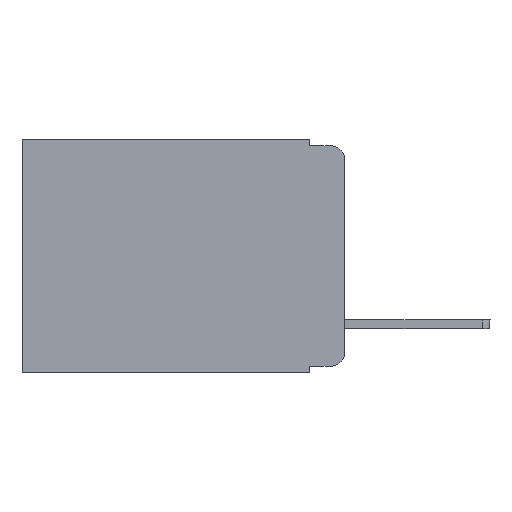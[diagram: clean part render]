
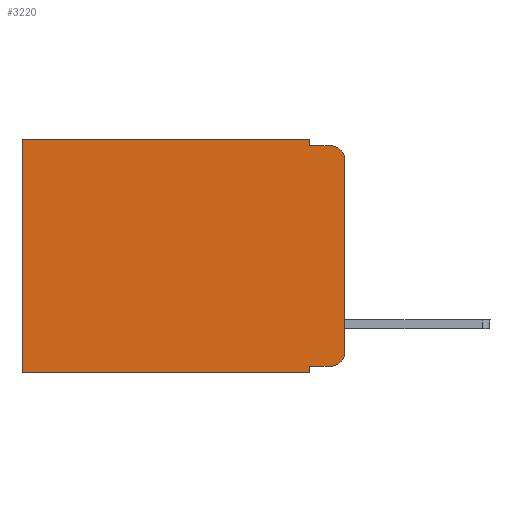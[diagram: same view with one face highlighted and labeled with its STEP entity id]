
A CAD part, left-side view. The second image highlights one B-rep face of the part: STEP entity #3220.
In plain terms, the highlighted planar face has unit normal (-1, 0, 0).
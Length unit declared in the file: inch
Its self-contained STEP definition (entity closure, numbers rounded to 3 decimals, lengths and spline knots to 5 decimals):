
#74 = VERTEX_POINT ( 'NONE', #2436 ) ;
#82 = ORIENTED_EDGE ( 'NONE', *, *, #1226, .T. ) ;
#198 = VERTEX_POINT ( 'NONE', #4855 ) ;
#212 = CARTESIAN_POINT ( 'NONE',  ( 0.298, 0., 0. ) ) ;
#234 = CIRCLE ( 'NONE', #6857, 0.02 ) ;
#612 = AXIS2_PLACEMENT_3D ( 'NONE', #3155, #5380, #3840 ) ;
#666 = EDGE_CURVE ( 'NONE', #4976, #74, #4478, .T. ) ;
#741 = EDGE_CURVE ( 'NONE', #7621, #8186, #6420, .T. ) ;
#754 = EDGE_CURVE ( 'NONE', #7621, #198, #1548, .T. ) ;
#815 = PLANE ( 'NONE',  #612 ) ;
#822 = VECTOR ( 'NONE', #1007, 39.37008 ) ;
#1007 = DIRECTION ( 'NONE',  ( 0., 0., -1. ) ) ;
#1194 = VECTOR ( 'NONE', #4541, 39.37008 ) ;
#1226 = EDGE_CURVE ( 'NONE', #8186, #9076, #8198, .T. ) ;
#1530 = VERTEX_POINT ( 'NONE', #3482 ) ;
#1548 = LINE ( 'NONE', #5641, #822 ) ;
#1569 = DIRECTION ( 'NONE',  ( 0., 0., -1. ) ) ;
#1584 = ORIENTED_EDGE ( 'NONE', *, *, #666, .F. ) ;
#1820 = EDGE_CURVE ( 'NONE', #5080, #1530, #2752, .T. ) ;
#1843 = VECTOR ( 'NONE', #6086, 39.37008 ) ;
#2134 = FACE_OUTER_BOUND ( 'NONE', #5461, .T. ) ;
#2274 = CARTESIAN_POINT ( 'NONE',  ( 0.298, 0.02, -0.313 ) ) ;
#2436 = CARTESIAN_POINT ( 'NONE',  ( 0.298, 0.051, -0.343 ) ) ;
#2606 = VECTOR ( 'NONE', #9206, 39.37008 ) ;
#2699 = ORIENTED_EDGE ( 'NONE', *, *, #4302, .F. ) ;
#2752 = CIRCLE ( 'NONE', #5102, 0.02 ) ;
#2829 = CARTESIAN_POINT ( 'NONE',  ( 0.298, 0.051, -0.333 ) ) ;
#2933 = CARTESIAN_POINT ( 'NONE',  ( 0.298, 0.051, -0.01 ) ) ;
#3155 = CARTESIAN_POINT ( 'NONE',  ( 0.298, 0., 0. ) ) ;
#3220 = ADVANCED_FACE ( 'NONE', ( #2134 ), #815, .F. ) ;
#3428 = CARTESIAN_POINT ( 'NONE',  ( 0.298, 0.473, 0. ) ) ;
#3482 = CARTESIAN_POINT ( 'NONE',  ( 0.298, 0., -0.313 ) ) ;
#3529 = CARTESIAN_POINT ( 'NONE',  ( 0.298, 0.02, -0.01 ) ) ;
#3718 = EDGE_CURVE ( 'NONE', #6842, #1530, #9592, .T. ) ;
#3840 = DIRECTION ( 'NONE',  ( 0., 0., -1. ) ) ;
#3881 = CARTESIAN_POINT ( 'NONE',  ( 0.298, 0.02, -0.03 ) ) ;
#4141 = ORIENTED_EDGE ( 'NONE', *, *, #1820, .T. ) ;
#4200 = ORIENTED_EDGE ( 'NONE', *, *, #741, .T. ) ;
#4302 = EDGE_CURVE ( 'NONE', #74, #9076, #6329, .T. ) ;
#4478 = LINE ( 'NONE', #9219, #8437 ) ;
#4519 = CARTESIAN_POINT ( 'NONE',  ( 0.298, 0.473, -0.343 ) ) ;
#4525 = DIRECTION ( 'NONE',  ( 0., 0., -1. ) ) ;
#4528 = VERTEX_POINT ( 'NONE', #3529 ) ;
#4541 = DIRECTION ( 'NONE',  ( 0., 0., -1. ) ) ;
#4617 = DIRECTION ( 'NONE',  ( 0., 0., -1. ) ) ;
#4644 = DIRECTION ( 'NONE',  ( -1., 0., 0. ) ) ;
#4675 = CARTESIAN_POINT ( 'NONE',  ( 0.298, 0.02, -0.333 ) ) ;
#4855 = CARTESIAN_POINT ( 'NONE',  ( 0.298, 0.051, -0.01 ) ) ;
#4976 = VERTEX_POINT ( 'NONE', #5300 ) ;
#5080 = VERTEX_POINT ( 'NONE', #4675 ) ;
#5102 = AXIS2_PLACEMENT_3D ( 'NONE', #2274, #7616, #4525 ) ;
#5136 = ORIENTED_EDGE ( 'NONE', *, *, #5707, .T. ) ;
#5300 = CARTESIAN_POINT ( 'NONE',  ( 0.298, 0.051, -0.333 ) ) ;
#5380 = DIRECTION ( 'NONE',  ( 1., 0., 0. ) ) ;
#5461 = EDGE_LOOP ( 'NONE', ( #8235, #5136, #7060, #6546, #4200, #82, #2699, #1584, #6085, #4141 ) ) ;
#5641 = CARTESIAN_POINT ( 'NONE',  ( 0.298, 0.051, 0. ) ) ;
#5707 = EDGE_CURVE ( 'NONE', #6842, #4528, #234, .T. ) ;
#6085 = ORIENTED_EDGE ( 'NONE', *, *, #8899, .T. ) ;
#6086 = DIRECTION ( 'NONE',  ( 0., 1., 0. ) ) ;
#6281 = CARTESIAN_POINT ( 'NONE',  ( 0.298, 0., -0.03 ) ) ;
#6329 = LINE ( 'NONE', #9150, #1843 ) ;
#6420 = LINE ( 'NONE', #212, #6767 ) ;
#6546 = ORIENTED_EDGE ( 'NONE', *, *, #754, .F. ) ;
#6583 = DIRECTION ( 'NONE',  ( 0., 0., -1. ) ) ;
#6767 = VECTOR ( 'NONE', #8669, 39.37008 ) ;
#6842 = VERTEX_POINT ( 'NONE', #6281 ) ;
#6857 = AXIS2_PLACEMENT_3D ( 'NONE', #3881, #4644, #4617 ) ;
#6970 = LINE ( 'NONE', #2933, #7951 ) ;
#7060 = ORIENTED_EDGE ( 'NONE', *, *, #7080, .F. ) ;
#7080 = EDGE_CURVE ( 'NONE', #198, #4528, #6970, .T. ) ;
#7430 = VECTOR ( 'NONE', #6583, 39.37008 ) ;
#7561 = LINE ( 'NONE', #2829, #2606 ) ;
#7601 = CARTESIAN_POINT ( 'NONE',  ( 0.298, 0.473, 0. ) ) ;
#7616 = DIRECTION ( 'NONE',  ( -1., 0., 0. ) ) ;
#7621 = VERTEX_POINT ( 'NONE', #9672 ) ;
#7951 = VECTOR ( 'NONE', #9120, 39.37008 ) ;
#8186 = VERTEX_POINT ( 'NONE', #3428 ) ;
#8198 = LINE ( 'NONE', #7601, #1194 ) ;
#8235 = ORIENTED_EDGE ( 'NONE', *, *, #3718, .F. ) ;
#8254 = CARTESIAN_POINT ( 'NONE',  ( 0.298, 0., 0. ) ) ;
#8437 = VECTOR ( 'NONE', #1569, 39.37008 ) ;
#8669 = DIRECTION ( 'NONE',  ( 0., 1., 0. ) ) ;
#8899 = EDGE_CURVE ( 'NONE', #4976, #5080, #7561, .T. ) ;
#9076 = VERTEX_POINT ( 'NONE', #4519 ) ;
#9120 = DIRECTION ( 'NONE',  ( 0., -1., 0. ) ) ;
#9150 = CARTESIAN_POINT ( 'NONE',  ( 0.298, 0., -0.343 ) ) ;
#9206 = DIRECTION ( 'NONE',  ( 0., -1., 0. ) ) ;
#9219 = CARTESIAN_POINT ( 'NONE',  ( 0.298, 0.051, 0. ) ) ;
#9592 = LINE ( 'NONE', #8254, #7430 ) ;
#9672 = CARTESIAN_POINT ( 'NONE',  ( 0.298, 0.051, 0. ) ) ;
